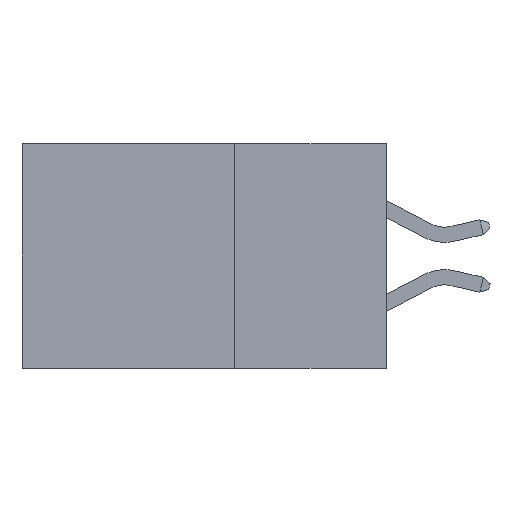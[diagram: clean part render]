
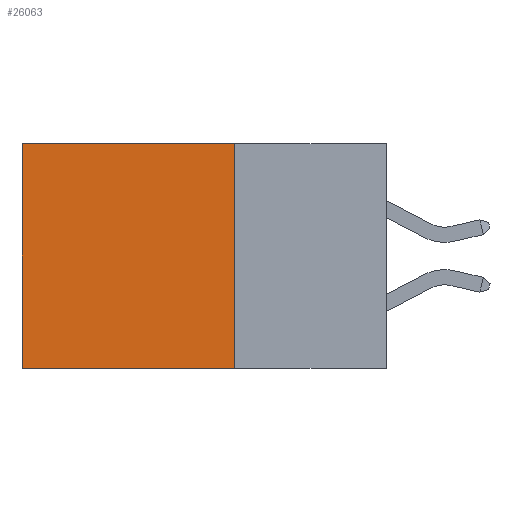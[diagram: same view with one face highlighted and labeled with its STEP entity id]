
A CAD part, left-side view. The second image highlights one B-rep face of the part: STEP entity #26063.
In plain terms, the highlighted planar face has unit normal (-1, 0, 0).
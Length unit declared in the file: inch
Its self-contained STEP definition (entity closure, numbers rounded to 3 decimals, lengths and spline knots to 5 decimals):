
#1174 = DIRECTION ( 'NONE',  ( 0., 0., -1. ) ) ;
#1520 = VECTOR ( 'NONE', #6200, 39.37008 ) ;
#3261 = DIRECTION ( 'NONE',  ( 1., 0., 0. ) ) ;
#4955 = PLANE ( 'NONE',  #19288 ) ;
#6200 = DIRECTION ( 'NONE',  ( 0., 1., 0. ) ) ;
#6700 = VECTOR ( 'NONE', #1174, 39.37008 ) ;
#7615 = FACE_OUTER_BOUND ( 'NONE', #23239, .T. ) ;
#7835 = DIRECTION ( 'NONE',  ( 0., 0., -1. ) ) ;
#8471 = LINE ( 'NONE', #15507, #1520 ) ;
#9177 = ORIENTED_EDGE ( 'NONE', *, *, #10072, .F. ) ;
#9790 = CARTESIAN_POINT ( 'NONE',  ( 0.298, 0.6, 0. ) ) ;
#10072 = EDGE_CURVE ( 'NONE', #23489, #13949, #22775, .T. ) ;
#10111 = CARTESIAN_POINT ( 'NONE',  ( 0.298, 0.25, -0.37 ) ) ;
#11031 = CARTESIAN_POINT ( 'NONE',  ( 0.298, 0.6, -0.37 ) ) ;
#11151 = EDGE_CURVE ( 'NONE', #13335, #23489, #28143, .T. ) ;
#12334 = CARTESIAN_POINT ( 'NONE',  ( 0.298, 0.25, 0. ) ) ;
#13335 = VERTEX_POINT ( 'NONE', #12334 ) ;
#13949 = VERTEX_POINT ( 'NONE', #11031 ) ;
#14895 = CARTESIAN_POINT ( 'NONE',  ( 0.298, 0.25, 0. ) ) ;
#15507 = CARTESIAN_POINT ( 'NONE',  ( 0.298, 0.25, 0. ) ) ;
#15756 = EDGE_CURVE ( 'NONE', #18347, #13949, #25166, .T. ) ;
#16041 = EDGE_CURVE ( 'NONE', #13335, #18347, #8471, .T. ) ;
#16805 = ORIENTED_EDGE ( 'NONE', *, *, #16041, .T. ) ;
#18347 = VERTEX_POINT ( 'NONE', #28529 ) ;
#19037 = VECTOR ( 'NONE', #7835, 39.37008 ) ;
#19288 = AXIS2_PLACEMENT_3D ( 'NONE', #14895, #3261, #23571 ) ;
#19362 = DIRECTION ( 'NONE',  ( 0., 1., 0. ) ) ;
#19479 = ORIENTED_EDGE ( 'NONE', *, *, #15756, .T. ) ;
#20495 = CARTESIAN_POINT ( 'NONE',  ( 0.298, 0.25, -0.37 ) ) ;
#22775 = LINE ( 'NONE', #10111, #25989 ) ;
#23239 = EDGE_LOOP ( 'NONE', ( #19479, #9177, #25068, #16805 ) ) ;
#23489 = VERTEX_POINT ( 'NONE', #20495 ) ;
#23571 = DIRECTION ( 'NONE',  ( 0., 0., -1. ) ) ;
#25068 = ORIENTED_EDGE ( 'NONE', *, *, #11151, .F. ) ;
#25166 = LINE ( 'NONE', #9790, #19037 ) ;
#25989 = VECTOR ( 'NONE', #19362, 39.37008 ) ;
#26063 = ADVANCED_FACE ( 'NONE', ( #7615 ), #4955, .F. ) ;
#28143 = LINE ( 'NONE', #29344, #6700 ) ;
#28529 = CARTESIAN_POINT ( 'NONE',  ( 0.298, 0.6, 0. ) ) ;
#29344 = CARTESIAN_POINT ( 'NONE',  ( 0.298, 0.25, 0. ) ) ;
